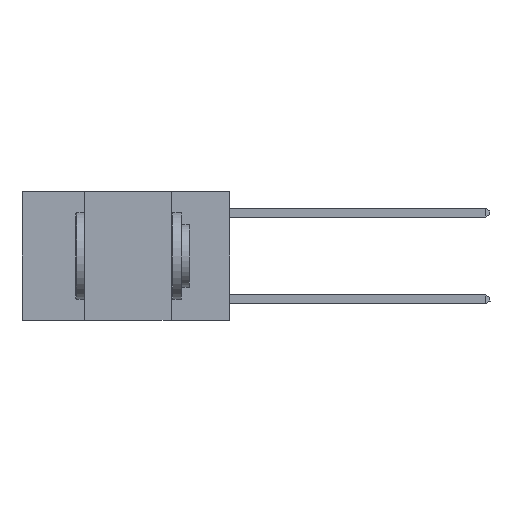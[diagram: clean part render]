
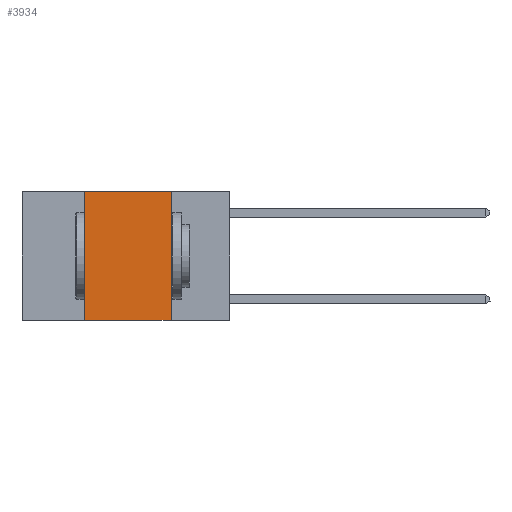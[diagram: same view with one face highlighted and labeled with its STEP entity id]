
A CAD part, left-side view. The second image highlights one B-rep face of the part: STEP entity #3934.
In plain terms, the highlighted planar face has unit normal (-1, 0, 0).
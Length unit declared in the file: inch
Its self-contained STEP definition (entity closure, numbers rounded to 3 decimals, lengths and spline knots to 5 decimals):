
#1628 = ORIENTED_EDGE ( 'NONE', *, *, #5569, .F. ) ;
#2762 = CARTESIAN_POINT ( 'NONE',  ( 0., 0.6, 0. ) ) ;
#2950 = EDGE_CURVE ( 'NONE', #22875, #8815, #15205, .T. ) ;
#3137 = CARTESIAN_POINT ( 'NONE',  ( 0., 0.17, -0.37 ) ) ;
#3326 = VECTOR ( 'NONE', #14253, 39.37008 ) ;
#3934 = ADVANCED_FACE ( 'NONE', ( #22598 ), #19679, .F. ) ;
#4131 = EDGE_CURVE ( 'NONE', #15428, #7235, #18377, .T. ) ;
#5074 = VECTOR ( 'NONE', #14826, 39.37008 ) ;
#5569 = EDGE_CURVE ( 'NONE', #8815, #7235, #10667, .T. ) ;
#5591 = LINE ( 'NONE', #23097, #10512 ) ;
#6311 = CARTESIAN_POINT ( 'NONE',  ( 0., 0.17, 0. ) ) ;
#6979 = DIRECTION ( 'NONE',  ( 1., 0., 0. ) ) ;
#7235 = VERTEX_POINT ( 'NONE', #3137 ) ;
#8354 = EDGE_CURVE ( 'NONE', #15428, #22875, #5591, .T. ) ;
#8815 = VERTEX_POINT ( 'NONE', #9631 ) ;
#9631 = CARTESIAN_POINT ( 'NONE',  ( 0., 0.17, 0. ) ) ;
#10512 = VECTOR ( 'NONE', #12521, 39.37008 ) ;
#10667 = LINE ( 'NONE', #6311, #5074 ) ;
#11896 = ORIENTED_EDGE ( 'NONE', *, *, #2950, .F. ) ;
#12379 = CARTESIAN_POINT ( 'NONE',  ( 0., 0.42, 0. ) ) ;
#12521 = DIRECTION ( 'NONE',  ( 0., 0., 1. ) ) ;
#13033 = ORIENTED_EDGE ( 'NONE', *, *, #4131, .T. ) ;
#13900 = ORIENTED_EDGE ( 'NONE', *, *, #8354, .F. ) ;
#14253 = DIRECTION ( 'NONE',  ( 0., -1., 0. ) ) ;
#14826 = DIRECTION ( 'NONE',  ( 0., 0., -1. ) ) ;
#15205 = LINE ( 'NONE', #18413, #3326 ) ;
#15428 = VERTEX_POINT ( 'NONE', #20405 ) ;
#15702 = EDGE_LOOP ( 'NONE', ( #1628, #11896, #13900, #13033 ) ) ;
#16044 = CARTESIAN_POINT ( 'NONE',  ( 0., 0.6, -0.37 ) ) ;
#18377 = LINE ( 'NONE', #16044, #23296 ) ;
#18413 = CARTESIAN_POINT ( 'NONE',  ( 0., 0.6, 0. ) ) ;
#19634 = AXIS2_PLACEMENT_3D ( 'NONE', #2762, #6979, #21775 ) ;
#19679 = PLANE ( 'NONE',  #19634 ) ;
#20405 = CARTESIAN_POINT ( 'NONE',  ( 0., 0.42, -0.37 ) ) ;
#21775 = DIRECTION ( 'NONE',  ( 0., 0., -1. ) ) ;
#22390 = DIRECTION ( 'NONE',  ( 0., -1., 0. ) ) ;
#22598 = FACE_OUTER_BOUND ( 'NONE', #15702, .T. ) ;
#22875 = VERTEX_POINT ( 'NONE', #12379 ) ;
#23097 = CARTESIAN_POINT ( 'NONE',  ( 0., 0.42, 0. ) ) ;
#23296 = VECTOR ( 'NONE', #22390, 39.37008 ) ;
